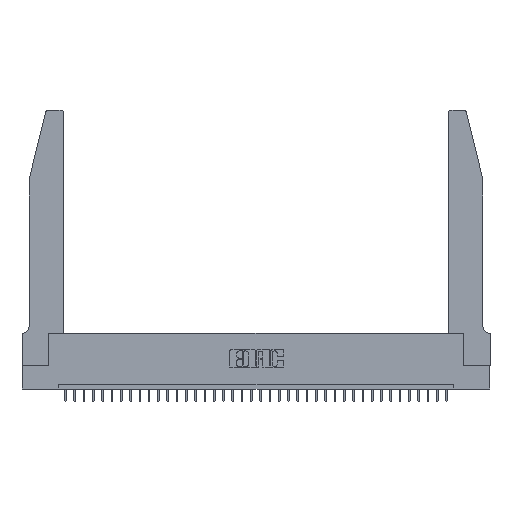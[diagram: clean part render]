
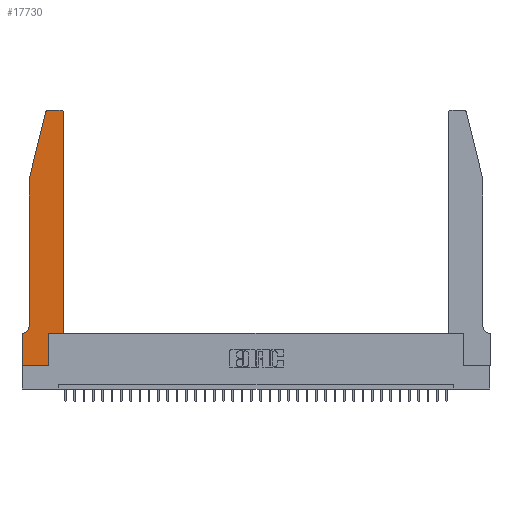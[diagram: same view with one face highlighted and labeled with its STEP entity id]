
A CAD part, top view. The second image highlights one B-rep face of the part: STEP entity #17730.
In plain terms, the highlighted planar face has unit normal (0, 0, 1).
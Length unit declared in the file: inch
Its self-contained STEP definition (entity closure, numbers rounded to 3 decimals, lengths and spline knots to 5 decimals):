
#291 = CARTESIAN_POINT ( 'NONE',  ( 0.0055, 0.35, 0.37 ) ) ;
#384 = VERTEX_POINT ( 'NONE', #21206 ) ;
#574 = CARTESIAN_POINT ( 'NONE',  ( 0.284, 2.75, 0.37 ) ) ;
#711 = VERTEX_POINT ( 'NONE', #574 ) ;
#1411 = EDGE_CURVE ( 'NONE', #12869, #20032, #20369, .T. ) ;
#2087 = AXIS2_PLACEMENT_3D ( 'NONE', #34351, #31762, #9051 ) ;
#2416 = EDGE_CURVE ( 'NONE', #21275, #16173, #12845, .T. ) ;
#2819 = EDGE_CURVE ( 'NONE', #384, #12869, #18464, .T. ) ;
#2820 = VECTOR ( 'NONE', #26865, 39.37008 ) ;
#3278 = DIRECTION ( 'NONE',  ( 0., 0., 1. ) ) ;
#3930 = DIRECTION ( 'NONE',  ( 1., 0., 0. ) ) ;
#3943 = AXIS2_PLACEMENT_3D ( 'NONE', #27951, #20490, #3930 ) ;
#4194 = CARTESIAN_POINT ( 'NONE',  ( 0.0755, 2., 0.37 ) ) ;
#4270 = VERTEX_POINT ( 'NONE', #17348 ) ;
#4599 = VECTOR ( 'NONE', #16405, 39.37008 ) ;
#4624 = VERTEX_POINT ( 'NONE', #14907 ) ;
#5586 = AXIS2_PLACEMENT_3D ( 'NONE', #31121, #3278, #8593 ) ;
#6797 = LINE ( 'NONE', #23569, #25058 ) ;
#7695 = VECTOR ( 'NONE', #30935, 39.37008 ) ;
#8098 = ORIENTED_EDGE ( 'NONE', *, *, #32023, .T. ) ;
#8593 = DIRECTION ( 'NONE',  ( 1., 0., 0. ) ) ;
#9051 = DIRECTION ( 'NONE',  ( 1., 0., 0. ) ) ;
#9095 = ORIENTED_EDGE ( 'NONE', *, *, #20714, .T. ) ;
#9479 = CIRCLE ( 'NONE', #21772, 0.07 ) ;
#9689 = CIRCLE ( 'NONE', #5586, 0.03 ) ;
#9973 = EDGE_CURVE ( 'NONE', #14112, #35369, #9479, .T. ) ;
#10245 = EDGE_CURVE ( 'NONE', #20032, #711, #15351, .T. ) ;
#10549 = EDGE_LOOP ( 'NONE', ( #32496, #16270, #21665, #29433, #29952, #8098, #21626, #9095, #10621, #13395, #31901, #25548 ) ) ;
#10621 = ORIENTED_EDGE ( 'NONE', *, *, #36122, .T. ) ;
#10911 = EDGE_CURVE ( 'NONE', #26441, #15507, #27418, .T. ) ;
#11031 = LINE ( 'NONE', #22274, #26313 ) ;
#12228 = DIRECTION ( 'NONE',  ( -1., 0., 0. ) ) ;
#12331 = DIRECTION ( 'NONE',  ( 1., 0., 0. ) ) ;
#12396 = VECTOR ( 'NONE', #12228, 39.37008 ) ;
#12845 = LINE ( 'NONE', #4194, #2820 ) ;
#12869 = VERTEX_POINT ( 'NONE', #25204 ) ;
#13395 = ORIENTED_EDGE ( 'NONE', *, *, #18133, .T. ) ;
#14091 = DIRECTION ( 'NONE',  ( 0., 0., -1. ) ) ;
#14112 = VERTEX_POINT ( 'NONE', #28514 ) ;
#14136 = CARTESIAN_POINT ( 'NONE',  ( 0., 0., 0.37 ) ) ;
#14614 = FACE_OUTER_BOUND ( 'NONE', #10549, .T. ) ;
#14907 = CARTESIAN_POINT ( 'NONE',  ( 0.2865, 0., 0.37 ) ) ;
#15183 = DIRECTION ( 'NONE',  ( 0., 1., 0. ) ) ;
#15351 = LINE ( 'NONE', #17916, #12396 ) ;
#15430 = EDGE_CURVE ( 'NONE', #711, #21275, #9689, .T. ) ;
#15507 = VERTEX_POINT ( 'NONE', #14136 ) ;
#16173 = VERTEX_POINT ( 'NONE', #28432 ) ;
#16270 = ORIENTED_EDGE ( 'NONE', *, *, #15430, .T. ) ;
#16405 = DIRECTION ( 'NONE',  ( 0., 1., 0. ) ) ;
#17348 = CARTESIAN_POINT ( 'NONE',  ( 0.2865, 0.35, 0.37 ) ) ;
#17730 = ADVANCED_FACE ( 'NONE', ( #14614 ), #23077, .T. ) ;
#17916 = CARTESIAN_POINT ( 'NONE',  ( 0.2605, 2.75, 0.37 ) ) ;
#18081 = VECTOR ( 'NONE', #27135, 39.37008 ) ;
#18133 = EDGE_CURVE ( 'NONE', #4270, #384, #6797, .T. ) ;
#18464 = LINE ( 'NONE', #32707, #29726 ) ;
#20032 = VERTEX_POINT ( 'NONE', #35210 ) ;
#20123 = EDGE_CURVE ( 'NONE', #16173, #14112, #11031, .T. ) ;
#20365 = CARTESIAN_POINT ( 'NONE',  ( 0.0755, 0.35, 0.37 ) ) ;
#20369 = CIRCLE ( 'NONE', #3943, 0.03 ) ;
#20444 = VECTOR ( 'NONE', #31289, 39.37008 ) ;
#20490 = DIRECTION ( 'NONE',  ( 0., 0., 1. ) ) ;
#20714 = EDGE_CURVE ( 'NONE', #15507, #4624, #30090, .T. ) ;
#20762 = CARTESIAN_POINT ( 'NONE',  ( 0.25487, 2.72718, 0.37 ) ) ;
#21206 = CARTESIAN_POINT ( 'NONE',  ( 0.4505, 0.35, 0.37 ) ) ;
#21275 = VERTEX_POINT ( 'NONE', #20762 ) ;
#21590 = CARTESIAN_POINT ( 'NONE',  ( 0., 0., 0.37 ) ) ;
#21626 = ORIENTED_EDGE ( 'NONE', *, *, #10911, .T. ) ;
#21665 = ORIENTED_EDGE ( 'NONE', *, *, #2416, .T. ) ;
#21772 = AXIS2_PLACEMENT_3D ( 'NONE', #22005, #14091, #33657 ) ;
#22005 = CARTESIAN_POINT ( 'NONE',  ( 0.0055, 0.42, 0.37 ) ) ;
#22052 = CARTESIAN_POINT ( 'NONE',  ( 0., 0., 0.37 ) ) ;
#22274 = CARTESIAN_POINT ( 'NONE',  ( 0.0755, 2., 0.37 ) ) ;
#23077 = PLANE ( 'NONE',  #2087 ) ;
#23569 = CARTESIAN_POINT ( 'NONE',  ( 0.4505, 0.35, 0.37 ) ) ;
#25058 = VECTOR ( 'NONE', #12331, 39.37008 ) ;
#25204 = CARTESIAN_POINT ( 'NONE',  ( 0.4505, 2.72, 0.37 ) ) ;
#25408 = DIRECTION ( 'NONE',  ( 0., -1., 0. ) ) ;
#25548 = ORIENTED_EDGE ( 'NONE', *, *, #1411, .T. ) ;
#26313 = VECTOR ( 'NONE', #25408, 39.37008 ) ;
#26441 = VERTEX_POINT ( 'NONE', #28602 ) ;
#26865 = DIRECTION ( 'NONE',  ( -0.239, -0.971, 0. ) ) ;
#27135 = DIRECTION ( 'NONE',  ( 1., 0., 0. ) ) ;
#27418 = LINE ( 'NONE', #22052, #7695 ) ;
#27951 = CARTESIAN_POINT ( 'NONE',  ( 0.4205, 2.72, 0.37 ) ) ;
#28432 = CARTESIAN_POINT ( 'NONE',  ( 0.0755, 2., 0.37 ) ) ;
#28514 = CARTESIAN_POINT ( 'NONE',  ( 0.0755, 0.42, 0.37 ) ) ;
#28602 = CARTESIAN_POINT ( 'NONE',  ( 0., 0.35, 0.37 ) ) ;
#29433 = ORIENTED_EDGE ( 'NONE', *, *, #20123, .T. ) ;
#29726 = VECTOR ( 'NONE', #15183, 39.37008 ) ;
#29952 = ORIENTED_EDGE ( 'NONE', *, *, #9973, .T. ) ;
#30090 = LINE ( 'NONE', #21590, #18081 ) ;
#30448 = CARTESIAN_POINT ( 'NONE',  ( 0.2865, 0.35, 0.37 ) ) ;
#30935 = DIRECTION ( 'NONE',  ( 0., -1., 0. ) ) ;
#31121 = CARTESIAN_POINT ( 'NONE',  ( 0.284, 2.72, 0.37 ) ) ;
#31289 = DIRECTION ( 'NONE',  ( -1., 0., 0. ) ) ;
#31657 = LINE ( 'NONE', #20365, #20444 ) ;
#31762 = DIRECTION ( 'NONE',  ( 0., 0., 1. ) ) ;
#31901 = ORIENTED_EDGE ( 'NONE', *, *, #2819, .T. ) ;
#32023 = EDGE_CURVE ( 'NONE', #35369, #26441, #31657, .T. ) ;
#32496 = ORIENTED_EDGE ( 'NONE', *, *, #10245, .T. ) ;
#32707 = CARTESIAN_POINT ( 'NONE',  ( 0.4505, 0.35, 0.37 ) ) ;
#33582 = LINE ( 'NONE', #30448, #4599 ) ;
#33657 = DIRECTION ( 'NONE',  ( -1., 0., 0. ) ) ;
#34351 = CARTESIAN_POINT ( 'NONE',  ( 0., 0.35, 0.37 ) ) ;
#35210 = CARTESIAN_POINT ( 'NONE',  ( 0.4205, 2.75, 0.37 ) ) ;
#35369 = VERTEX_POINT ( 'NONE', #291 ) ;
#36122 = EDGE_CURVE ( 'NONE', #4624, #4270, #33582, .T. ) ;
